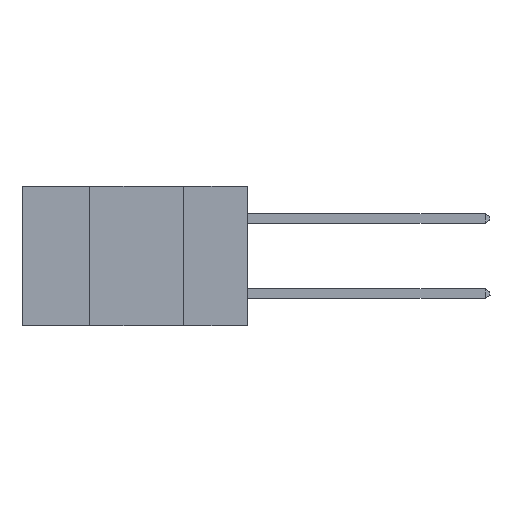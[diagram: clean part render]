
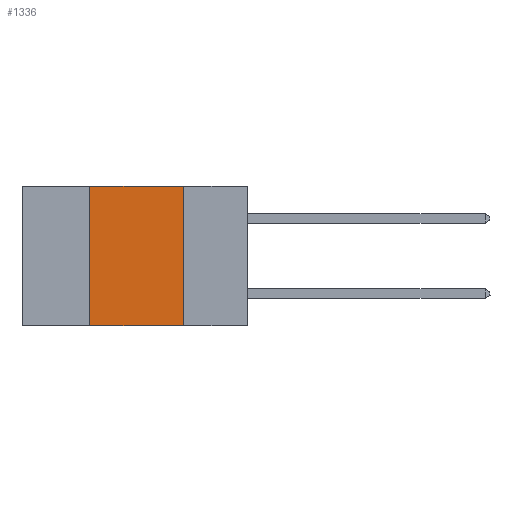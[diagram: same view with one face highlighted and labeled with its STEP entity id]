
A CAD part, left-side view. The second image highlights one B-rep face of the part: STEP entity #1336.
In plain terms, the highlighted planar face has unit normal (-1, 0, 0).
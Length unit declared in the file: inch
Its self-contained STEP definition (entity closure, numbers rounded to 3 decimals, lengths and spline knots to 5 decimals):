
#529 = CARTESIAN_POINT ( 'NONE',  ( 0., 0.6, -0.37 ) ) ;
#824 = DIRECTION ( 'NONE',  ( 1., 0., 0. ) ) ;
#1102 = ORIENTED_EDGE ( 'NONE', *, *, #7989, .F. ) ;
#1336 = ADVANCED_FACE ( 'NONE', ( #14483 ), #17843, .F. ) ;
#1433 = DIRECTION ( 'NONE',  ( 0., 0., 1. ) ) ;
#1775 = AXIS2_PLACEMENT_3D ( 'NONE', #2268, #824, #15088 ) ;
#2268 = CARTESIAN_POINT ( 'NONE',  ( 0., 0.6, 0. ) ) ;
#2274 = CARTESIAN_POINT ( 'NONE',  ( 0., 0.17, -0.37 ) ) ;
#3057 = CARTESIAN_POINT ( 'NONE',  ( 0., 0.42, 0. ) ) ;
#3324 = VERTEX_POINT ( 'NONE', #5302 ) ;
#3952 = VECTOR ( 'NONE', #11431, 39.37008 ) ;
#4097 = CARTESIAN_POINT ( 'NONE',  ( 0., 0.42, 0. ) ) ;
#4242 = ORIENTED_EDGE ( 'NONE', *, *, #13013, .F. ) ;
#4829 = VECTOR ( 'NONE', #1433, 39.37008 ) ;
#5302 = CARTESIAN_POINT ( 'NONE',  ( 0., 0.42, -0.37 ) ) ;
#6648 = VECTOR ( 'NONE', #12044, 39.37008 ) ;
#7009 = EDGE_CURVE ( 'NONE', #18180, #14538, #16029, .T. ) ;
#7989 = EDGE_CURVE ( 'NONE', #14538, #9227, #9790, .T. ) ;
#8555 = CARTESIAN_POINT ( 'NONE',  ( 0., 0.17, 0. ) ) ;
#8737 = VECTOR ( 'NONE', #14654, 39.37008 ) ;
#8896 = LINE ( 'NONE', #4097, #4829 ) ;
#9227 = VERTEX_POINT ( 'NONE', #2274 ) ;
#9790 = LINE ( 'NONE', #8555, #3952 ) ;
#10346 = EDGE_LOOP ( 'NONE', ( #1102, #16700, #4242, #18313 ) ) ;
#11431 = DIRECTION ( 'NONE',  ( 0., 0., -1. ) ) ;
#12044 = DIRECTION ( 'NONE',  ( 0., -1., 0. ) ) ;
#13013 = EDGE_CURVE ( 'NONE', #3324, #18180, #8896, .T. ) ;
#13250 = CARTESIAN_POINT ( 'NONE',  ( 0., 0.6, 0. ) ) ;
#13334 = LINE ( 'NONE', #529, #6648 ) ;
#13734 = EDGE_CURVE ( 'NONE', #3324, #9227, #13334, .T. ) ;
#14451 = CARTESIAN_POINT ( 'NONE',  ( 0., 0.17, 0. ) ) ;
#14483 = FACE_OUTER_BOUND ( 'NONE', #10346, .T. ) ;
#14538 = VERTEX_POINT ( 'NONE', #14451 ) ;
#14654 = DIRECTION ( 'NONE',  ( 0., -1., 0. ) ) ;
#15088 = DIRECTION ( 'NONE',  ( 0., 0., -1. ) ) ;
#16029 = LINE ( 'NONE', #13250, #8737 ) ;
#16700 = ORIENTED_EDGE ( 'NONE', *, *, #7009, .F. ) ;
#17843 = PLANE ( 'NONE',  #1775 ) ;
#18180 = VERTEX_POINT ( 'NONE', #3057 ) ;
#18313 = ORIENTED_EDGE ( 'NONE', *, *, #13734, .T. ) ;
